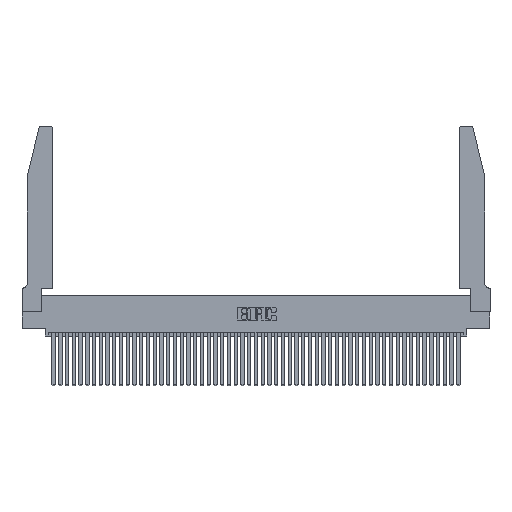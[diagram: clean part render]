
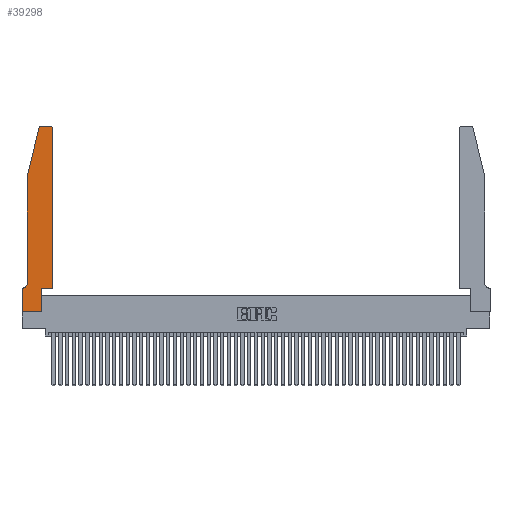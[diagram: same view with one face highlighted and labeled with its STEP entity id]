
A CAD part, top view. The second image highlights one B-rep face of the part: STEP entity #39298.
In plain terms, the highlighted planar face has unit normal (0, 0, 1).
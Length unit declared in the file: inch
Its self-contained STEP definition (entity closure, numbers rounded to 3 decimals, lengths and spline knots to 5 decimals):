
#750 = LINE ( 'NONE', #16939, #9793 ) ;
#1568 = EDGE_CURVE ( 'NONE', #17330, #43021, #15703, .T. ) ;
#1917 = DIRECTION ( 'NONE',  ( -1., 0., 0. ) ) ;
#2154 = CARTESIAN_POINT ( 'NONE',  ( 0., 0., 0.37 ) ) ;
#2616 = DIRECTION ( 'NONE',  ( 0., 0., 1. ) ) ;
#2797 = VERTEX_POINT ( 'NONE', #29245 ) ;
#3886 = CARTESIAN_POINT ( 'NONE',  ( 0., 0., 0.37 ) ) ;
#4702 = VECTOR ( 'NONE', #42299, 39.37008 ) ;
#5594 = VECTOR ( 'NONE', #29465, 39.37008 ) ;
#5659 = VERTEX_POINT ( 'NONE', #31760 ) ;
#5853 = LINE ( 'NONE', #10321, #36718 ) ;
#5899 = DIRECTION ( 'NONE',  ( 0., 0., 1. ) ) ;
#5936 = VECTOR ( 'NONE', #16398, 39.37008 ) ;
#6944 = CARTESIAN_POINT ( 'NONE',  ( 0.0755, 2., 0.37 ) ) ;
#7152 = LINE ( 'NONE', #12474, #5936 ) ;
#7480 = CARTESIAN_POINT ( 'NONE',  ( 0.0755, 2., 0.37 ) ) ;
#8602 = EDGE_CURVE ( 'NONE', #5659, #46561, #12178, .T. ) ;
#8897 = EDGE_CURVE ( 'NONE', #10650, #22810, #9022, .T. ) ;
#9022 = LINE ( 'NONE', #3886, #28491 ) ;
#9793 = VECTOR ( 'NONE', #35825, 39.37008 ) ;
#10096 = EDGE_CURVE ( 'NONE', #43021, #16983, #15085, .T. ) ;
#10321 = CARTESIAN_POINT ( 'NONE',  ( 0.4505, 0.35, 0.37 ) ) ;
#10650 = VERTEX_POINT ( 'NONE', #37354 ) ;
#11447 = ORIENTED_EDGE ( 'NONE', *, *, #50002, .T. ) ;
#11621 = CARTESIAN_POINT ( 'NONE',  ( 0.25487, 2.72718, 0.37 ) ) ;
#12178 = LINE ( 'NONE', #21751, #42954 ) ;
#12474 = CARTESIAN_POINT ( 'NONE',  ( 0.2605, 2.75, 0.37 ) ) ;
#12910 = VERTEX_POINT ( 'NONE', #45162 ) ;
#13340 = ORIENTED_EDGE ( 'NONE', *, *, #41212, .T. ) ;
#13749 = AXIS2_PLACEMENT_3D ( 'NONE', #37811, #14781, #41686 ) ;
#14125 = AXIS2_PLACEMENT_3D ( 'NONE', #29157, #5899, #33012 ) ;
#14492 = VECTOR ( 'NONE', #49292, 39.37008 ) ;
#14781 = DIRECTION ( 'NONE',  ( 0., 0., 1. ) ) ;
#15085 = LINE ( 'NONE', #7480, #4702 ) ;
#15703 = LINE ( 'NONE', #6944, #14492 ) ;
#16286 = EDGE_CURVE ( 'NONE', #46561, #2797, #35567, .T. ) ;
#16366 = ORIENTED_EDGE ( 'NONE', *, *, #43962, .T. ) ;
#16398 = DIRECTION ( 'NONE',  ( -1., 0., 0. ) ) ;
#16939 = CARTESIAN_POINT ( 'NONE',  ( 0.0755, 0.35, 0.37 ) ) ;
#16983 = VERTEX_POINT ( 'NONE', #17633 ) ;
#17330 = VERTEX_POINT ( 'NONE', #11621 ) ;
#17633 = CARTESIAN_POINT ( 'NONE',  ( 0.0755, 0.42, 0.37 ) ) ;
#18201 = ORIENTED_EDGE ( 'NONE', *, *, #8602, .T. ) ;
#18307 = VECTOR ( 'NONE', #40875, 39.37008 ) ;
#19539 = DIRECTION ( 'NONE',  ( 0., -1., 0. ) ) ;
#19928 = CIRCLE ( 'NONE', #30399, 0.07 ) ;
#20021 = ORIENTED_EDGE ( 'NONE', *, *, #20355, .T. ) ;
#20355 = EDGE_CURVE ( 'NONE', #12910, #10650, #750, .T. ) ;
#21747 = CARTESIAN_POINT ( 'NONE',  ( 0.2865, 0., 0.37 ) ) ;
#21751 = CARTESIAN_POINT ( 'NONE',  ( 0.4505, 0.35, 0.37 ) ) ;
#21841 = ORIENTED_EDGE ( 'NONE', *, *, #16286, .T. ) ;
#22024 = CARTESIAN_POINT ( 'NONE',  ( 0., 0.35, 0.37 ) ) ;
#22395 = VERTEX_POINT ( 'NONE', #38939 ) ;
#22473 = EDGE_CURVE ( 'NONE', #2797, #22395, #7152, .T. ) ;
#22810 = VERTEX_POINT ( 'NONE', #36837 ) ;
#23656 = ORIENTED_EDGE ( 'NONE', *, *, #45165, .T. ) ;
#24257 = EDGE_LOOP ( 'NONE', ( #41011, #11447, #44614, #25434, #16366, #20021, #42884, #13340, #23656, #37440, #18201, #21841 ) ) ;
#25221 = DIRECTION ( 'NONE',  ( 0., 0., -1. ) ) ;
#25434 = ORIENTED_EDGE ( 'NONE', *, *, #10096, .T. ) ;
#25591 = CARTESIAN_POINT ( 'NONE',  ( 0.2865, 0.35, 0.37 ) ) ;
#25636 = DIRECTION ( 'NONE',  ( 0., 1., 0. ) ) ;
#28491 = VECTOR ( 'NONE', #19539, 39.37008 ) ;
#29157 = CARTESIAN_POINT ( 'NONE',  ( 0.4205, 2.72, 0.37 ) ) ;
#29245 = CARTESIAN_POINT ( 'NONE',  ( 0.4205, 2.75, 0.37 ) ) ;
#29465 = DIRECTION ( 'NONE',  ( 0., 1., 0. ) ) ;
#29772 = DIRECTION ( 'NONE',  ( 1., 0., 0. ) ) ;
#30399 = AXIS2_PLACEMENT_3D ( 'NONE', #48177, #25221, #1917 ) ;
#31760 = CARTESIAN_POINT ( 'NONE',  ( 0.4505, 0.35, 0.37 ) ) ;
#32359 = VERTEX_POINT ( 'NONE', #21747 ) ;
#33012 = DIRECTION ( 'NONE',  ( 1., 0., 0. ) ) ;
#33561 = DIRECTION ( 'NONE',  ( 1., 0., 0. ) ) ;
#34892 = CIRCLE ( 'NONE', #13749, 0.03 ) ;
#35239 = VERTEX_POINT ( 'NONE', #39995 ) ;
#35567 = CIRCLE ( 'NONE', #14125, 0.03 ) ;
#35825 = DIRECTION ( 'NONE',  ( -1., 0., 0. ) ) ;
#36481 = LINE ( 'NONE', #25591, #5594 ) ;
#36718 = VECTOR ( 'NONE', #33561, 39.37008 ) ;
#36837 = CARTESIAN_POINT ( 'NONE',  ( 0., 0., 0.37 ) ) ;
#37354 = CARTESIAN_POINT ( 'NONE',  ( 0., 0.35, 0.37 ) ) ;
#37440 = ORIENTED_EDGE ( 'NONE', *, *, #49263, .T. ) ;
#37811 = CARTESIAN_POINT ( 'NONE',  ( 0.284, 2.72, 0.37 ) ) ;
#38939 = CARTESIAN_POINT ( 'NONE',  ( 0.284, 2.75, 0.37 ) ) ;
#39298 = ADVANCED_FACE ( 'NONE', ( #41358 ), #48859, .T. ) ;
#39995 = CARTESIAN_POINT ( 'NONE',  ( 0.2865, 0.35, 0.37 ) ) ;
#40875 = DIRECTION ( 'NONE',  ( 1., 0., 0. ) ) ;
#41011 = ORIENTED_EDGE ( 'NONE', *, *, #22473, .T. ) ;
#41212 = EDGE_CURVE ( 'NONE', #22810, #32359, #48955, .T. ) ;
#41358 = FACE_OUTER_BOUND ( 'NONE', #24257, .T. ) ;
#41686 = DIRECTION ( 'NONE',  ( 1., 0., 0. ) ) ;
#42299 = DIRECTION ( 'NONE',  ( 0., -1., 0. ) ) ;
#42884 = ORIENTED_EDGE ( 'NONE', *, *, #8897, .T. ) ;
#42954 = VECTOR ( 'NONE', #25636, 39.37008 ) ;
#43021 = VERTEX_POINT ( 'NONE', #48102 ) ;
#43962 = EDGE_CURVE ( 'NONE', #16983, #12910, #19928, .T. ) ;
#44614 = ORIENTED_EDGE ( 'NONE', *, *, #1568, .T. ) ;
#44946 = CARTESIAN_POINT ( 'NONE',  ( 0.4505, 2.72, 0.37 ) ) ;
#45162 = CARTESIAN_POINT ( 'NONE',  ( 0.0055, 0.35, 0.37 ) ) ;
#45165 = EDGE_CURVE ( 'NONE', #32359, #35239, #36481, .T. ) ;
#46314 = AXIS2_PLACEMENT_3D ( 'NONE', #22024, #2616, #29772 ) ;
#46561 = VERTEX_POINT ( 'NONE', #44946 ) ;
#48102 = CARTESIAN_POINT ( 'NONE',  ( 0.0755, 2., 0.37 ) ) ;
#48177 = CARTESIAN_POINT ( 'NONE',  ( 0.0055, 0.42, 0.37 ) ) ;
#48859 = PLANE ( 'NONE',  #46314 ) ;
#48955 = LINE ( 'NONE', #2154, #18307 ) ;
#49263 = EDGE_CURVE ( 'NONE', #35239, #5659, #5853, .T. ) ;
#49292 = DIRECTION ( 'NONE',  ( -0.239, -0.971, 0. ) ) ;
#50002 = EDGE_CURVE ( 'NONE', #22395, #17330, #34892, .T. ) ;
